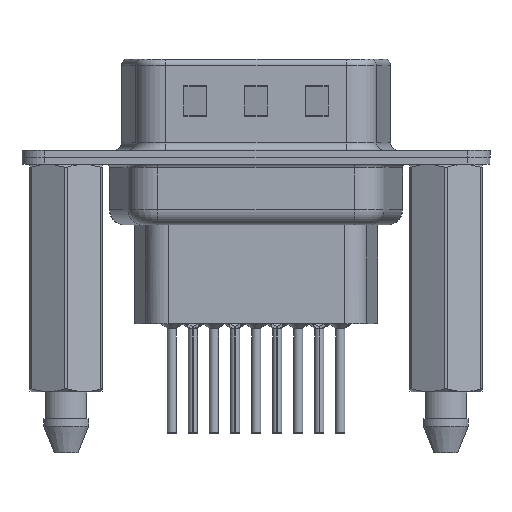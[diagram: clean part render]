
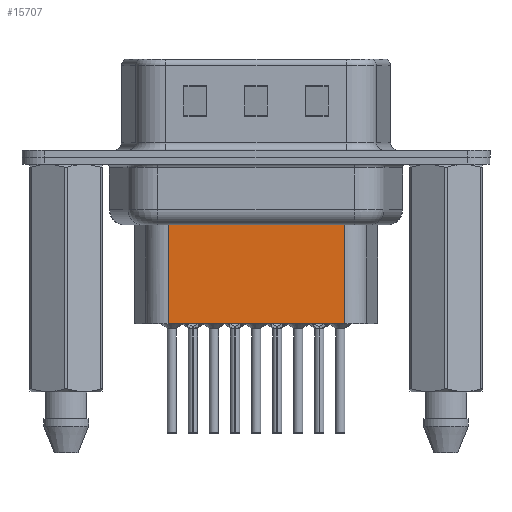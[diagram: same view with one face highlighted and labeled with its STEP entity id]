
A CAD part, front view. The second image highlights one B-rep face of the part: STEP entity #15707.
In plain terms, the highlighted planar face has unit normal (0, -1, 0).
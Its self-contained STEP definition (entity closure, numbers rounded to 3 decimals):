
#301 = DIRECTION ( 'NONE',  ( -1., 0., 0. ) ) ;
#511 = VECTOR ( 'NONE', #5784, 1000. ) ;
#805 = CARTESIAN_POINT ( 'NONE',  ( 18.294, -3.5, -4.097 ) ) ;
#1021 = CARTESIAN_POINT ( 'NONE',  ( 18.294, -3.5, -10.95 ) ) ;
#2084 = LINE ( 'NONE', #7249, #14119 ) ;
#3537 = ORIENTED_EDGE ( 'NONE', *, *, #16328, .F. ) ;
#3568 = ORIENTED_EDGE ( 'NONE', *, *, #20028, .F. ) ;
#4163 = VERTEX_POINT ( 'NONE', #805 ) ;
#4500 = PLANE ( 'NONE',  #16417 ) ;
#5038 = EDGE_LOOP ( 'NONE', ( #3568, #14945, #21143, #3537 ) ) ;
#5284 = VERTEX_POINT ( 'NONE', #15087 ) ;
#5771 = CARTESIAN_POINT ( 'NONE',  ( 6.706, -3.5, -4.097 ) ) ;
#5784 = DIRECTION ( 'NONE',  ( -1., 0., 0. ) ) ;
#5816 = DIRECTION ( 'NONE',  ( 1., 0., 0. ) ) ;
#6017 = DIRECTION ( 'NONE',  ( 0., -1., 0. ) ) ;
#7249 = CARTESIAN_POINT ( 'NONE',  ( 18.294, -3.5, -3.1 ) ) ;
#8187 = VECTOR ( 'NONE', #301, 1000. ) ;
#13029 = CARTESIAN_POINT ( 'NONE',  ( 6.706, -3.5, -10.95 ) ) ;
#13571 = EDGE_CURVE ( 'NONE', #4163, #18265, #13969, .T. ) ;
#13643 = VERTEX_POINT ( 'NONE', #1021 ) ;
#13969 = LINE ( 'NONE', #20511, #511 ) ;
#14119 = VECTOR ( 'NONE', #20277, 1000. ) ;
#14945 = ORIENTED_EDGE ( 'NONE', *, *, #13571, .T. ) ;
#15087 = CARTESIAN_POINT ( 'NONE',  ( 6.706, -3.5, -10.95 ) ) ;
#15428 = VECTOR ( 'NONE', #19345, 1000. ) ;
#15707 = ADVANCED_FACE ( 'NONE', ( #19149 ), #4500, .T. ) ;
#16328 = EDGE_CURVE ( 'NONE', #13643, #5284, #16574, .T. ) ;
#16417 = AXIS2_PLACEMENT_3D ( 'NONE', #17541, #6017, #5816 ) ;
#16574 = LINE ( 'NONE', #13029, #8187 ) ;
#17541 = CARTESIAN_POINT ( 'NONE',  ( 6.706, -3.5, -3.1 ) ) ;
#17728 = LINE ( 'NONE', #19031, #15428 ) ;
#17939 = EDGE_CURVE ( 'NONE', #18265, #5284, #17728, .T. ) ;
#18265 = VERTEX_POINT ( 'NONE', #5771 ) ;
#19031 = CARTESIAN_POINT ( 'NONE',  ( 6.706, -3.5, -3.1 ) ) ;
#19149 = FACE_OUTER_BOUND ( 'NONE', #5038, .T. ) ;
#19345 = DIRECTION ( 'NONE',  ( 0., 0., -1. ) ) ;
#20028 = EDGE_CURVE ( 'NONE', #4163, #13643, #2084, .T. ) ;
#20277 = DIRECTION ( 'NONE',  ( 0., 0., -1. ) ) ;
#20511 = CARTESIAN_POINT ( 'NONE',  ( 6.459, -3.5, -4.097 ) ) ;
#21143 = ORIENTED_EDGE ( 'NONE', *, *, #17939, .T. ) ;
